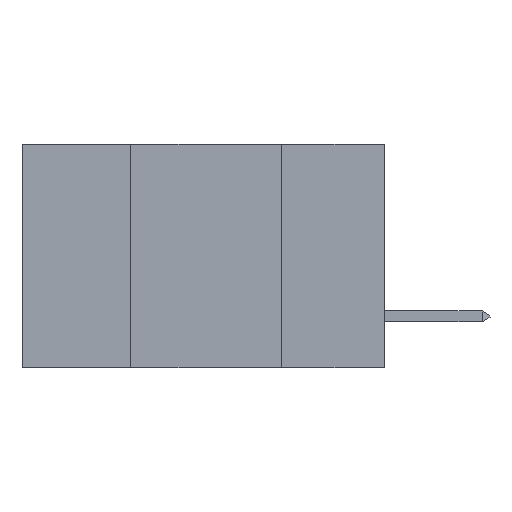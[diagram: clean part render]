
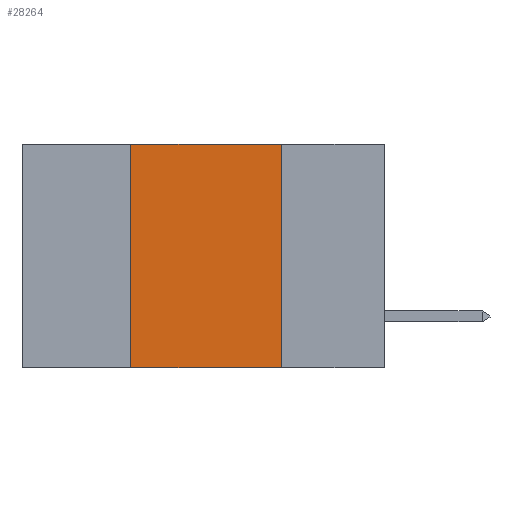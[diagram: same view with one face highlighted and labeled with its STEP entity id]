
A CAD part, left-side view. The second image highlights one B-rep face of the part: STEP entity #28264.
In plain terms, the highlighted planar face has unit normal (-1, 0, 0).
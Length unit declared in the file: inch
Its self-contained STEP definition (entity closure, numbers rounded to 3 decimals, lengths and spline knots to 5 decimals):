
#1250 = CARTESIAN_POINT ( 'NONE',  ( 0., 0.17, 0. ) ) ;
#1287 = VERTEX_POINT ( 'NONE', #9821 ) ;
#1598 = LINE ( 'NONE', #18449, #26363 ) ;
#1711 = EDGE_CURVE ( 'NONE', #10576, #1287, #18649, .T. ) ;
#4254 = AXIS2_PLACEMENT_3D ( 'NONE', #11368, #28075, #13737 ) ;
#6611 = ORIENTED_EDGE ( 'NONE', *, *, #1711, .F. ) ;
#8348 = LINE ( 'NONE', #23378, #13903 ) ;
#8917 = EDGE_LOOP ( 'NONE', ( #6611, #13708, #27171, #21552 ) ) ;
#9153 = FACE_OUTER_BOUND ( 'NONE', #8917, .T. ) ;
#9821 = CARTESIAN_POINT ( 'NONE',  ( 0., 0.17, -0.37 ) ) ;
#10576 = VERTEX_POINT ( 'NONE', #1250 ) ;
#11368 = CARTESIAN_POINT ( 'NONE',  ( 0., 0.6, 0. ) ) ;
#11943 = CARTESIAN_POINT ( 'NONE',  ( 0., 0.17, 0. ) ) ;
#12300 = VECTOR ( 'NONE', #31118, 39.37008 ) ;
#13708 = ORIENTED_EDGE ( 'NONE', *, *, #20669, .F. ) ;
#13737 = DIRECTION ( 'NONE',  ( 0., 0., -1. ) ) ;
#13878 = DIRECTION ( 'NONE',  ( 0., 0., 1. ) ) ;
#13903 = VECTOR ( 'NONE', #13878, 39.37008 ) ;
#17772 = EDGE_CURVE ( 'NONE', #21950, #20372, #8348, .T. ) ;
#18449 = CARTESIAN_POINT ( 'NONE',  ( 0., 0.6, -0.37 ) ) ;
#18649 = LINE ( 'NONE', #11943, #12300 ) ;
#19962 = CARTESIAN_POINT ( 'NONE',  ( 0., 0.6, 0. ) ) ;
#20372 = VERTEX_POINT ( 'NONE', #21306 ) ;
#20413 = CARTESIAN_POINT ( 'NONE',  ( 0., 0.42, -0.37 ) ) ;
#20669 = EDGE_CURVE ( 'NONE', #20372, #10576, #23786, .T. ) ;
#21306 = CARTESIAN_POINT ( 'NONE',  ( 0., 0.42, 0. ) ) ;
#21552 = ORIENTED_EDGE ( 'NONE', *, *, #27179, .T. ) ;
#21950 = VERTEX_POINT ( 'NONE', #20413 ) ;
#22339 = DIRECTION ( 'NONE',  ( 0., -1., 0. ) ) ;
#23052 = VECTOR ( 'NONE', #22339, 39.37008 ) ;
#23220 = DIRECTION ( 'NONE',  ( 0., -1., 0. ) ) ;
#23378 = CARTESIAN_POINT ( 'NONE',  ( 0., 0.42, 0. ) ) ;
#23786 = LINE ( 'NONE', #19962, #23052 ) ;
#25631 = PLANE ( 'NONE',  #4254 ) ;
#26363 = VECTOR ( 'NONE', #23220, 39.37008 ) ;
#27171 = ORIENTED_EDGE ( 'NONE', *, *, #17772, .F. ) ;
#27179 = EDGE_CURVE ( 'NONE', #21950, #1287, #1598, .T. ) ;
#28075 = DIRECTION ( 'NONE',  ( 1., 0., 0. ) ) ;
#28264 = ADVANCED_FACE ( 'NONE', ( #9153 ), #25631, .F. ) ;
#31118 = DIRECTION ( 'NONE',  ( 0., 0., -1. ) ) ;
